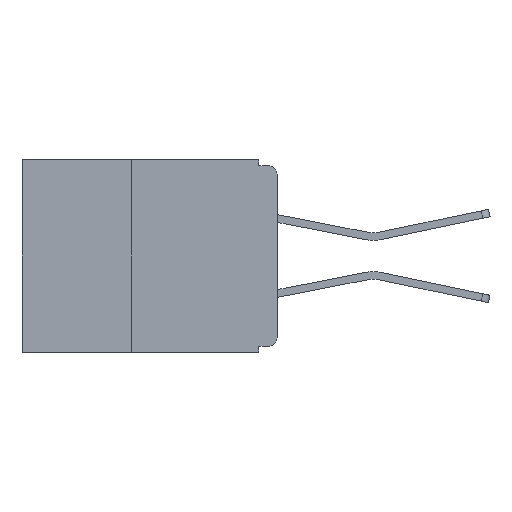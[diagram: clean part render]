
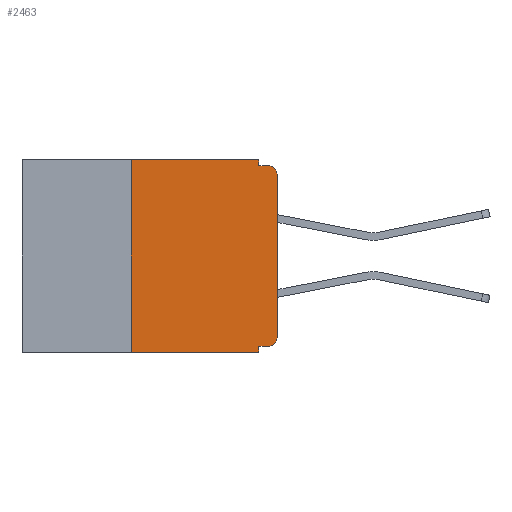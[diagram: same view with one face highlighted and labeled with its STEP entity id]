
A CAD part, left-side view. The second image highlights one B-rep face of the part: STEP entity #2463.
In plain terms, the highlighted planar face has unit normal (-1, 0, 0).
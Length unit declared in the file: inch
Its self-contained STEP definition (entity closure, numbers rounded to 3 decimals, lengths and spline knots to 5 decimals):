
#17 = DIRECTION ( 'NONE',  ( 0., 0., 1. ) ) ;
#39 = CARTESIAN_POINT ( 'NONE',  ( 0., 0., -0.01 ) ) ;
#124 = DIRECTION ( 'NONE',  ( 0., 0., -1. ) ) ;
#407 = CARTESIAN_POINT ( 'NONE',  ( 0., 0.031, -0.32 ) ) ;
#649 = CARTESIAN_POINT ( 'NONE',  ( 0., 0.015, -0.305 ) ) ;
#668 = CARTESIAN_POINT ( 'NONE',  ( 0., 0.25, -0.33 ) ) ;
#910 = VECTOR ( 'NONE', #1042, 39.37008 ) ;
#1042 = DIRECTION ( 'NONE',  ( 0., 0., -1. ) ) ;
#1165 = DIRECTION ( 'NONE',  ( 0., 0., 1. ) ) ;
#1375 = ORIENTED_EDGE ( 'NONE', *, *, #1756, .F. ) ;
#1389 = PLANE ( 'NONE',  #12824 ) ;
#1400 = DIRECTION ( 'NONE',  ( 1., 0., 0. ) ) ;
#1756 = EDGE_CURVE ( 'NONE', #11926, #2930, #10550, .T. ) ;
#1769 = DIRECTION ( 'NONE',  ( 0., 0., -1. ) ) ;
#2003 = AXIS2_PLACEMENT_3D ( 'NONE', #13205, #6580, #14311 ) ;
#2078 = EDGE_CURVE ( 'NONE', #11368, #11926, #12571, .T. ) ;
#2097 = EDGE_CURVE ( 'NONE', #5841, #4183, #12226, .T. ) ;
#2272 = CARTESIAN_POINT ( 'NONE',  ( 0., 0.437, 0. ) ) ;
#2463 = ADVANCED_FACE ( 'NONE', ( #5069 ), #1389, .F. ) ;
#2525 = VERTEX_POINT ( 'NONE', #13648 ) ;
#2930 = VERTEX_POINT ( 'NONE', #5982 ) ;
#2931 = VECTOR ( 'NONE', #4540, 39.37008 ) ;
#3020 = LINE ( 'NONE', #10612, #14157 ) ;
#3235 = ORIENTED_EDGE ( 'NONE', *, *, #2078, .F. ) ;
#3503 = CARTESIAN_POINT ( 'NONE',  ( 0., 0., -0.305 ) ) ;
#3676 = VECTOR ( 'NONE', #17, 39.37008 ) ;
#4183 = VERTEX_POINT ( 'NONE', #9904 ) ;
#4277 = CIRCLE ( 'NONE', #7087, 0.015 ) ;
#4356 = ORIENTED_EDGE ( 'NONE', *, *, #5365, .F. ) ;
#4372 = ORIENTED_EDGE ( 'NONE', *, *, #10389, .F. ) ;
#4540 = DIRECTION ( 'NONE',  ( 0., 0., -1. ) ) ;
#4927 = VERTEX_POINT ( 'NONE', #3503 ) ;
#5063 = VERTEX_POINT ( 'NONE', #11574 ) ;
#5069 = FACE_OUTER_BOUND ( 'NONE', #6438, .T. ) ;
#5212 = EDGE_CURVE ( 'NONE', #2525, #4927, #4277, .T. ) ;
#5365 = EDGE_CURVE ( 'NONE', #2525, #12271, #10972, .T. ) ;
#5438 = EDGE_CURVE ( 'NONE', #12271, #5063, #6922, .T. ) ;
#5806 = EDGE_CURVE ( 'NONE', #11368, #5063, #3020, .T. ) ;
#5841 = VERTEX_POINT ( 'NONE', #8382 ) ;
#5855 = ORIENTED_EDGE ( 'NONE', *, *, #2097, .F. ) ;
#5953 = LINE ( 'NONE', #10143, #2931 ) ;
#5982 = CARTESIAN_POINT ( 'NONE',  ( 0., 0.031, 0. ) ) ;
#6438 = EDGE_LOOP ( 'NONE', ( #7321, #7342, #5855, #4372, #1375, #3235, #8271, #10442, #4356, #11134 ) ) ;
#6580 = DIRECTION ( 'NONE',  ( -1., 0., 0. ) ) ;
#6581 = DIRECTION ( 'NONE',  ( 0., 1., 0. ) ) ;
#6922 = LINE ( 'NONE', #12231, #910 ) ;
#7087 = AXIS2_PLACEMENT_3D ( 'NONE', #649, #8537, #1769 ) ;
#7218 = DIRECTION ( 'NONE',  ( 0., -1., 0. ) ) ;
#7321 = ORIENTED_EDGE ( 'NONE', *, *, #10955, .T. ) ;
#7342 = ORIENTED_EDGE ( 'NONE', *, *, #8753, .T. ) ;
#7538 = VECTOR ( 'NONE', #9575, 39.37008 ) ;
#7670 = VECTOR ( 'NONE', #1165, 39.37008 ) ;
#7746 = CIRCLE ( 'NONE', #2003, 0.015 ) ;
#8271 = ORIENTED_EDGE ( 'NONE', *, *, #5806, .T. ) ;
#8382 = CARTESIAN_POINT ( 'NONE',  ( 0., 0.031, -0.01 ) ) ;
#8492 = CARTESIAN_POINT ( 'NONE',  ( 0., 0.25, -0.33 ) ) ;
#8537 = DIRECTION ( 'NONE',  ( -1., 0., 0. ) ) ;
#8753 = EDGE_CURVE ( 'NONE', #13198, #4183, #7746, .T. ) ;
#9281 = VECTOR ( 'NONE', #14232, 39.37008 ) ;
#9575 = DIRECTION ( 'NONE',  ( 0., -1., 0. ) ) ;
#9677 = CARTESIAN_POINT ( 'NONE',  ( 0., 0.437, 0. ) ) ;
#9866 = CARTESIAN_POINT ( 'NONE',  ( 0., 0.25, 0. ) ) ;
#9904 = CARTESIAN_POINT ( 'NONE',  ( 0., 0.015, -0.01 ) ) ;
#10143 = CARTESIAN_POINT ( 'NONE',  ( 0., 0.031, 0. ) ) ;
#10389 = EDGE_CURVE ( 'NONE', #2930, #5841, #5953, .T. ) ;
#10442 = ORIENTED_EDGE ( 'NONE', *, *, #5438, .F. ) ;
#10550 = LINE ( 'NONE', #9677, #7538 ) ;
#10612 = CARTESIAN_POINT ( 'NONE',  ( 0., 0.437, -0.33 ) ) ;
#10630 = VECTOR ( 'NONE', #6581, 39.37008 ) ;
#10676 = LINE ( 'NONE', #11267, #7670 ) ;
#10955 = EDGE_CURVE ( 'NONE', #4927, #13198, #10676, .T. ) ;
#10972 = LINE ( 'NONE', #13206, #10630 ) ;
#11134 = ORIENTED_EDGE ( 'NONE', *, *, #5212, .T. ) ;
#11267 = CARTESIAN_POINT ( 'NONE',  ( 0., 0., 0. ) ) ;
#11368 = VERTEX_POINT ( 'NONE', #8492 ) ;
#11574 = CARTESIAN_POINT ( 'NONE',  ( 0., 0.031, -0.33 ) ) ;
#11926 = VERTEX_POINT ( 'NONE', #9866 ) ;
#12226 = LINE ( 'NONE', #39, #9281 ) ;
#12231 = CARTESIAN_POINT ( 'NONE',  ( 0., 0.031, -0.33 ) ) ;
#12271 = VERTEX_POINT ( 'NONE', #407 ) ;
#12571 = LINE ( 'NONE', #668, #3676 ) ;
#12824 = AXIS2_PLACEMENT_3D ( 'NONE', #2272, #1400, #124 ) ;
#13198 = VERTEX_POINT ( 'NONE', #13284 ) ;
#13205 = CARTESIAN_POINT ( 'NONE',  ( 0., 0.015, -0.025 ) ) ;
#13206 = CARTESIAN_POINT ( 'NONE',  ( 0., 0., -0.32 ) ) ;
#13284 = CARTESIAN_POINT ( 'NONE',  ( 0., 0., -0.025 ) ) ;
#13648 = CARTESIAN_POINT ( 'NONE',  ( 0., 0.015, -0.32 ) ) ;
#14157 = VECTOR ( 'NONE', #7218, 39.37008 ) ;
#14232 = DIRECTION ( 'NONE',  ( 0., -1., 0. ) ) ;
#14311 = DIRECTION ( 'NONE',  ( 0., 0., -1. ) ) ;
